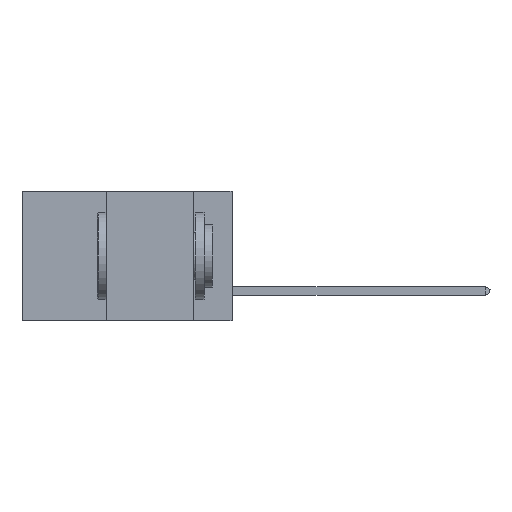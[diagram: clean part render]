
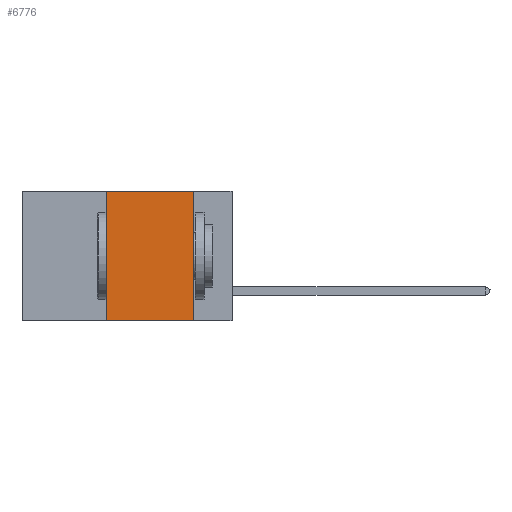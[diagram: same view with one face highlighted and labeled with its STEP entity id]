
A CAD part, left-side view. The second image highlights one B-rep face of the part: STEP entity #6776.
In plain terms, the highlighted planar face has unit normal (-1, 0, 0).
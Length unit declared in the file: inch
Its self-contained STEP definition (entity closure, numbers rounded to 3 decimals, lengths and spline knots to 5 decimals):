
#33 = LINE ( 'NONE', #28301, #23502 ) ;
#3042 = EDGE_LOOP ( 'NONE', ( #20601, #7735, #5814, #38103 ) ) ;
#3095 = DIRECTION ( 'NONE',  ( 0., 0., -1. ) ) ;
#5287 = DIRECTION ( 'NONE',  ( 0., -1., 0. ) ) ;
#5814 = ORIENTED_EDGE ( 'NONE', *, *, #24897, .F. ) ;
#5904 = VERTEX_POINT ( 'NONE', #42294 ) ;
#6307 = VECTOR ( 'NONE', #5287, 39.37008 ) ;
#6776 = ADVANCED_FACE ( 'NONE', ( #25710 ), #39122, .F. ) ;
#7735 = ORIENTED_EDGE ( 'NONE', *, *, #7826, .F. ) ;
#7826 = EDGE_CURVE ( 'NONE', #25230, #17758, #33, .T. ) ;
#8292 = CARTESIAN_POINT ( 'NONE',  ( 0., 0.11, 0. ) ) ;
#9439 = CARTESIAN_POINT ( 'NONE',  ( 0., 0.36, 0. ) ) ;
#10762 = LINE ( 'NONE', #36659, #14372 ) ;
#11305 = DIRECTION ( 'NONE',  ( 0., 0., 1. ) ) ;
#14372 = VECTOR ( 'NONE', #11305, 39.37008 ) ;
#15118 = AXIS2_PLACEMENT_3D ( 'NONE', #23494, #39325, #3095 ) ;
#16138 = DIRECTION ( 'NONE',  ( 0., -1., 0. ) ) ;
#16486 = EDGE_CURVE ( 'NONE', #5904, #37277, #28843, .T. ) ;
#17331 = VECTOR ( 'NONE', #17359, 39.37008 ) ;
#17359 = DIRECTION ( 'NONE',  ( 0., 0., -1. ) ) ;
#17758 = VERTEX_POINT ( 'NONE', #8292 ) ;
#17857 = LINE ( 'NONE', #26426, #17331 ) ;
#20601 = ORIENTED_EDGE ( 'NONE', *, *, #33799, .F. ) ;
#23494 = CARTESIAN_POINT ( 'NONE',  ( 0., 0.6, 0. ) ) ;
#23502 = VECTOR ( 'NONE', #16138, 39.37008 ) ;
#23526 = CARTESIAN_POINT ( 'NONE',  ( 0., 0.11, -0.37 ) ) ;
#24897 = EDGE_CURVE ( 'NONE', #5904, #25230, #10762, .T. ) ;
#25230 = VERTEX_POINT ( 'NONE', #9439 ) ;
#25301 = CARTESIAN_POINT ( 'NONE',  ( 0., 0.6, -0.37 ) ) ;
#25710 = FACE_OUTER_BOUND ( 'NONE', #3042, .T. ) ;
#26426 = CARTESIAN_POINT ( 'NONE',  ( 0., 0.11, 0. ) ) ;
#28301 = CARTESIAN_POINT ( 'NONE',  ( 0., 0.6, 0. ) ) ;
#28843 = LINE ( 'NONE', #25301, #6307 ) ;
#33799 = EDGE_CURVE ( 'NONE', #17758, #37277, #17857, .T. ) ;
#36659 = CARTESIAN_POINT ( 'NONE',  ( 0., 0.36, 0. ) ) ;
#37277 = VERTEX_POINT ( 'NONE', #23526 ) ;
#38103 = ORIENTED_EDGE ( 'NONE', *, *, #16486, .T. ) ;
#39122 = PLANE ( 'NONE',  #15118 ) ;
#39325 = DIRECTION ( 'NONE',  ( 1., 0., 0. ) ) ;
#42294 = CARTESIAN_POINT ( 'NONE',  ( 0., 0.36, -0.37 ) ) ;
